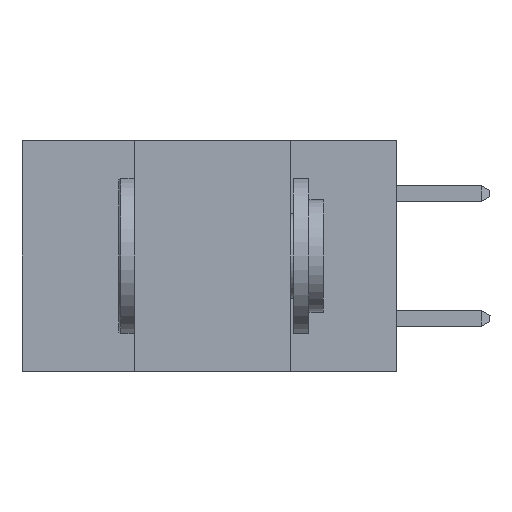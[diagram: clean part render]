
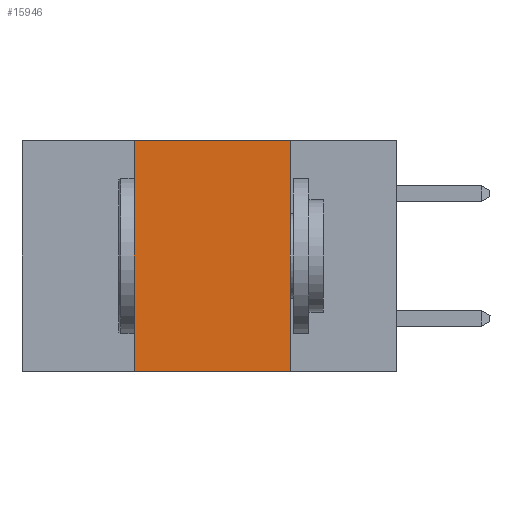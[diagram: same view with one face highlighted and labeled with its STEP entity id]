
A CAD part, left-side view. The second image highlights one B-rep face of the part: STEP entity #15946.
In plain terms, the highlighted planar face has unit normal (-1, 0, 0).
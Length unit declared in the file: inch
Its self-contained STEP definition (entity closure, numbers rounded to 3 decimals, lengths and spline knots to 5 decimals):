
#1119 = EDGE_CURVE ( 'NONE', #27402, #1611, #28626, .T. ) ;
#1611 = VERTEX_POINT ( 'NONE', #12769 ) ;
#2461 = VECTOR ( 'NONE', #5976, 39.37008 ) ;
#2844 = LINE ( 'NONE', #4184, #27972 ) ;
#2940 = ORIENTED_EDGE ( 'NONE', *, *, #21166, .F. ) ;
#3473 = ORIENTED_EDGE ( 'NONE', *, *, #6757, .F. ) ;
#4184 = CARTESIAN_POINT ( 'NONE',  ( 0., 0.6, -0.37 ) ) ;
#4672 = VERTEX_POINT ( 'NONE', #6741 ) ;
#4767 = ORIENTED_EDGE ( 'NONE', *, *, #20724, .T. ) ;
#5375 = CARTESIAN_POINT ( 'NONE',  ( 0., 0.42, 0. ) ) ;
#5878 = AXIS2_PLACEMENT_3D ( 'NONE', #8563, #20140, #13321 ) ;
#5976 = DIRECTION ( 'NONE',  ( 0., 0., -1. ) ) ;
#6741 = CARTESIAN_POINT ( 'NONE',  ( 0., 0.42, 0. ) ) ;
#6757 = EDGE_CURVE ( 'NONE', #4672, #27402, #11208, .T. ) ;
#8472 = LINE ( 'NONE', #5375, #12999 ) ;
#8563 = CARTESIAN_POINT ( 'NONE',  ( 0., 0.6, 0. ) ) ;
#10981 = DIRECTION ( 'NONE',  ( 0., -1., 0. ) ) ;
#11208 = LINE ( 'NONE', #23970, #16496 ) ;
#11943 = CARTESIAN_POINT ( 'NONE',  ( 0., 0.17, 0. ) ) ;
#12283 = CARTESIAN_POINT ( 'NONE',  ( 0., 0.42, -0.37 ) ) ;
#12769 = CARTESIAN_POINT ( 'NONE',  ( 0., 0.17, -0.37 ) ) ;
#12999 = VECTOR ( 'NONE', #25427, 39.37008 ) ;
#13321 = DIRECTION ( 'NONE',  ( 0., 0., -1. ) ) ;
#14512 = CARTESIAN_POINT ( 'NONE',  ( 0., 0.17, 0. ) ) ;
#15392 = FACE_OUTER_BOUND ( 'NONE', #28772, .T. ) ;
#15946 = ADVANCED_FACE ( 'NONE', ( #15392 ), #26275, .F. ) ;
#16496 = VECTOR ( 'NONE', #10981, 39.37008 ) ;
#17605 = DIRECTION ( 'NONE',  ( 0., -1., 0. ) ) ;
#18962 = VERTEX_POINT ( 'NONE', #12283 ) ;
#20140 = DIRECTION ( 'NONE',  ( 1., 0., 0. ) ) ;
#20724 = EDGE_CURVE ( 'NONE', #18962, #1611, #2844, .T. ) ;
#21166 = EDGE_CURVE ( 'NONE', #18962, #4672, #8472, .T. ) ;
#23970 = CARTESIAN_POINT ( 'NONE',  ( 0., 0.6, 0. ) ) ;
#25427 = DIRECTION ( 'NONE',  ( 0., 0., 1. ) ) ;
#26275 = PLANE ( 'NONE',  #5878 ) ;
#27402 = VERTEX_POINT ( 'NONE', #11943 ) ;
#27972 = VECTOR ( 'NONE', #17605, 39.37008 ) ;
#28388 = ORIENTED_EDGE ( 'NONE', *, *, #1119, .F. ) ;
#28626 = LINE ( 'NONE', #14512, #2461 ) ;
#28772 = EDGE_LOOP ( 'NONE', ( #28388, #3473, #2940, #4767 ) ) ;
